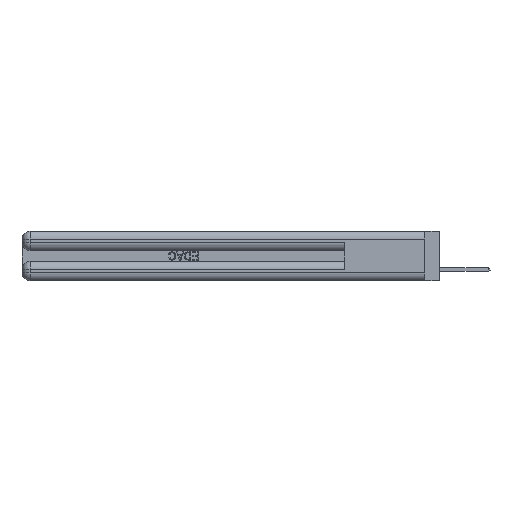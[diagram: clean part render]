
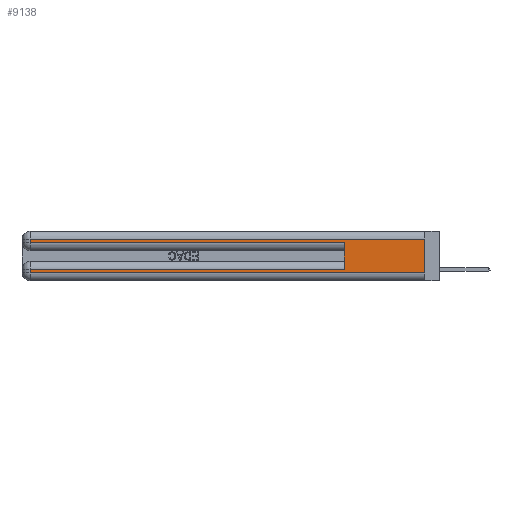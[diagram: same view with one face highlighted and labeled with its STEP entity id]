
A CAD part, left-side view. The second image highlights one B-rep face of the part: STEP entity #9138.
In plain terms, the highlighted planar face has unit normal (-1, 0, 0).
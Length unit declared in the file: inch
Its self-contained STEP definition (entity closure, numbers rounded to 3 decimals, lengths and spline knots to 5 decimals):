
#1364 = EDGE_CURVE ( 'NONE', #36994, #41420, #13804, .T. ) ;
#1541 = CARTESIAN_POINT ( 'NONE',  ( 0., 0., 0.37 ) ) ;
#1683 = LINE ( 'NONE', #8798, #36049 ) ;
#1717 = VERTEX_POINT ( 'NONE', #8737 ) ;
#2630 = VECTOR ( 'NONE', #12214, 39.37008 ) ;
#3196 = LINE ( 'NONE', #8844, #2630 ) ;
#3590 = LINE ( 'NONE', #14916, #27403 ) ;
#4669 = CARTESIAN_POINT ( 'NONE',  ( 0., 0.6, 0.085 ) ) ;
#5479 = AXIS2_PLACEMENT_3D ( 'NONE', #23748, #26464, #13125 ) ;
#7107 = CARTESIAN_POINT ( 'NONE',  ( 0., 0., 0.085 ) ) ;
#7134 = VECTOR ( 'NONE', #16970, 39.37008 ) ;
#7767 = EDGE_CURVE ( 'NONE', #41070, #13476, #3590, .T. ) ;
#7908 = EDGE_CURVE ( 'NONE', #33887, #43624, #30536, .T. ) ;
#8121 = DIRECTION ( 'NONE',  ( 0., 0., 1. ) ) ;
#8737 = CARTESIAN_POINT ( 'NONE',  ( 0., 2.94, 0.085 ) ) ;
#8798 = CARTESIAN_POINT ( 'NONE',  ( 0., 2.94, 0.37 ) ) ;
#8844 = CARTESIAN_POINT ( 'NONE',  ( 0., 2.94, 0.37 ) ) ;
#9138 = ADVANCED_FACE ( 'NONE', ( #10415 ), #23606, .F. ) ;
#10047 = EDGE_CURVE ( 'NONE', #33887, #41420, #33062, .T. ) ;
#10415 = FACE_OUTER_BOUND ( 'NONE', #17705, .T. ) ;
#10940 = VECTOR ( 'NONE', #22468, 39.37008 ) ;
#11269 = ORIENTED_EDGE ( 'NONE', *, *, #7908, .T. ) ;
#11889 = EDGE_CURVE ( 'NONE', #1717, #36994, #3196, .T. ) ;
#11953 = VERTEX_POINT ( 'NONE', #21117 ) ;
#12018 = DIRECTION ( 'NONE',  ( 0., -1., 0. ) ) ;
#12214 = DIRECTION ( 'NONE',  ( 0., 0., -1. ) ) ;
#12419 = ORIENTED_EDGE ( 'NONE', *, *, #1364, .T. ) ;
#13078 = ORIENTED_EDGE ( 'NONE', *, *, #10047, .F. ) ;
#13125 = DIRECTION ( 'NONE',  ( 0., 0., -1. ) ) ;
#13476 = VERTEX_POINT ( 'NONE', #33540 ) ;
#13804 = LINE ( 'NONE', #29055, #14321 ) ;
#14321 = VECTOR ( 'NONE', #12018, 39.37008 ) ;
#14916 = CARTESIAN_POINT ( 'NONE',  ( 0., 0.6, 0.145 ) ) ;
#15495 = CARTESIAN_POINT ( 'NONE',  ( 0., 0., 0.31 ) ) ;
#16970 = DIRECTION ( 'NONE',  ( 0., -1., 0. ) ) ;
#17597 = ORIENTED_EDGE ( 'NONE', *, *, #27732, .T. ) ;
#17705 = EDGE_LOOP ( 'NONE', ( #13078, #11269, #17597, #30303, #24399, #37844, #21329, #12419 ) ) ;
#18370 = EDGE_CURVE ( 'NONE', #41070, #1717, #18681, .T. ) ;
#18681 = LINE ( 'NONE', #7107, #39785 ) ;
#21027 = DIRECTION ( 'NONE',  ( 0., 1., 0. ) ) ;
#21117 = CARTESIAN_POINT ( 'NONE',  ( 0., 2.94, 0.285 ) ) ;
#21329 = ORIENTED_EDGE ( 'NONE', *, *, #11889, .T. ) ;
#22468 = DIRECTION ( 'NONE',  ( 0., 1., 0. ) ) ;
#23524 = VECTOR ( 'NONE', #31818, 39.37008 ) ;
#23606 = PLANE ( 'NONE',  #5479 ) ;
#23748 = CARTESIAN_POINT ( 'NONE',  ( 0., 0., 0.37 ) ) ;
#24399 = ORIENTED_EDGE ( 'NONE', *, *, #7767, .F. ) ;
#25055 = DIRECTION ( 'NONE',  ( 0., 0., -1. ) ) ;
#25070 = CARTESIAN_POINT ( 'NONE',  ( 0., 0., 0.31 ) ) ;
#26464 = DIRECTION ( 'NONE',  ( 1., 0., 0. ) ) ;
#27403 = VECTOR ( 'NONE', #8121, 39.37008 ) ;
#27732 = EDGE_CURVE ( 'NONE', #43624, #11953, #1683, .T. ) ;
#29055 = CARTESIAN_POINT ( 'NONE',  ( 0., 0., 0.06 ) ) ;
#30303 = ORIENTED_EDGE ( 'NONE', *, *, #39085, .T. ) ;
#30352 = CARTESIAN_POINT ( 'NONE',  ( 0., 2.94, 0.06 ) ) ;
#30536 = LINE ( 'NONE', #15495, #10940 ) ;
#31818 = DIRECTION ( 'NONE',  ( 0., 0., -1. ) ) ;
#33062 = LINE ( 'NONE', #1541, #23524 ) ;
#33458 = CARTESIAN_POINT ( 'NONE',  ( 0., 0., 0.06 ) ) ;
#33540 = CARTESIAN_POINT ( 'NONE',  ( 0., 0.6, 0.285 ) ) ;
#33887 = VERTEX_POINT ( 'NONE', #25070 ) ;
#35126 = LINE ( 'NONE', #37185, #7134 ) ;
#36049 = VECTOR ( 'NONE', #25055, 39.37008 ) ;
#36994 = VERTEX_POINT ( 'NONE', #30352 ) ;
#37185 = CARTESIAN_POINT ( 'NONE',  ( 0., 0., 0.285 ) ) ;
#37844 = ORIENTED_EDGE ( 'NONE', *, *, #18370, .T. ) ;
#38563 = CARTESIAN_POINT ( 'NONE',  ( 0., 2.94, 0.31 ) ) ;
#39085 = EDGE_CURVE ( 'NONE', #11953, #13476, #35126, .T. ) ;
#39785 = VECTOR ( 'NONE', #21027, 39.37008 ) ;
#41070 = VERTEX_POINT ( 'NONE', #4669 ) ;
#41420 = VERTEX_POINT ( 'NONE', #33458 ) ;
#43624 = VERTEX_POINT ( 'NONE', #38563 ) ;
